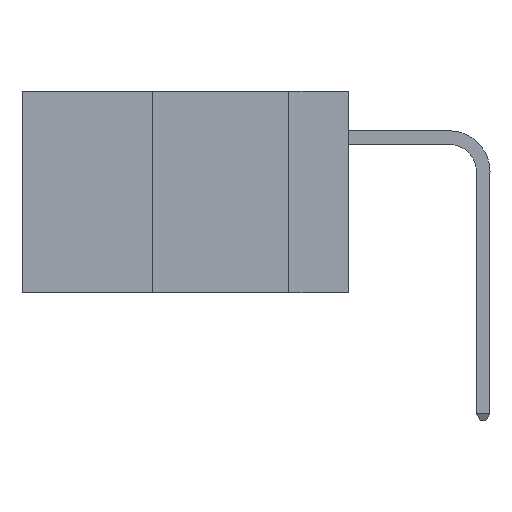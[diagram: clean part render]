
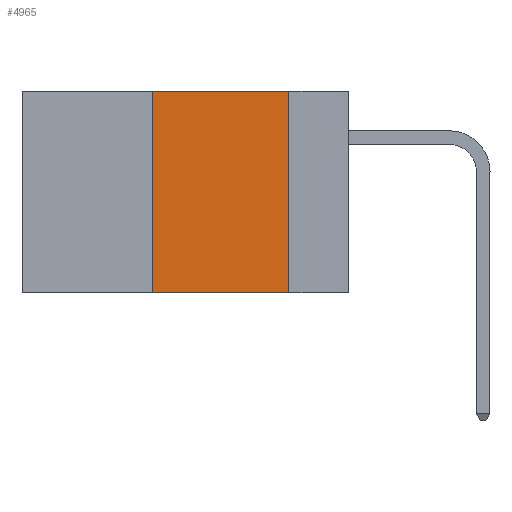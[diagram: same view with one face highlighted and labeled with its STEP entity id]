
A CAD part, left-side view. The second image highlights one B-rep face of the part: STEP entity #4965.
In plain terms, the highlighted planar face has unit normal (-1, 0, 0).
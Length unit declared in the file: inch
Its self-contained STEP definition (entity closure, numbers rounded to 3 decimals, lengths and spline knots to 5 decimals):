
#364 = EDGE_CURVE ( 'NONE', #6327, #7623, #7117, .T. ) ;
#445 = LINE ( 'NONE', #7259, #2283 ) ;
#888 = VECTOR ( 'NONE', #7565, 39.37008 ) ;
#1232 = PLANE ( 'NONE',  #2368 ) ;
#1266 = ORIENTED_EDGE ( 'NONE', *, *, #3956, .F. ) ;
#1365 = EDGE_CURVE ( 'NONE', #6327, #9292, #6985, .T. ) ;
#2129 = DIRECTION ( 'NONE',  ( 1., 0., 0. ) ) ;
#2200 = CARTESIAN_POINT ( 'NONE',  ( 0., 0.36, 0. ) ) ;
#2283 = VECTOR ( 'NONE', #10680, 39.37008 ) ;
#2368 = AXIS2_PLACEMENT_3D ( 'NONE', #7469, #2129, #8333 ) ;
#3110 = CARTESIAN_POINT ( 'NONE',  ( 0., 0.36, 0. ) ) ;
#3817 = DIRECTION ( 'NONE',  ( 0., -1., 0. ) ) ;
#3914 = ORIENTED_EDGE ( 'NONE', *, *, #1365, .F. ) ;
#3925 = ORIENTED_EDGE ( 'NONE', *, *, #9059, .F. ) ;
#3956 = EDGE_CURVE ( 'NONE', #9292, #4129, #8002, .T. ) ;
#4004 = CARTESIAN_POINT ( 'NONE',  ( 0., 0.6, 0. ) ) ;
#4129 = VERTEX_POINT ( 'NONE', #5207 ) ;
#4965 = ADVANCED_FACE ( 'NONE', ( #8970 ), #1232, .F. ) ;
#5207 = CARTESIAN_POINT ( 'NONE',  ( 0., 0.11, 0. ) ) ;
#5246 = EDGE_LOOP ( 'NONE', ( #3925, #1266, #3914, #5788 ) ) ;
#5788 = ORIENTED_EDGE ( 'NONE', *, *, #364, .T. ) ;
#6327 = VERTEX_POINT ( 'NONE', #9562 ) ;
#6985 = LINE ( 'NONE', #2200, #11247 ) ;
#7117 = LINE ( 'NONE', #8646, #11382 ) ;
#7259 = CARTESIAN_POINT ( 'NONE',  ( 0., 0.11, 0. ) ) ;
#7469 = CARTESIAN_POINT ( 'NONE',  ( 0., 0.6, 0. ) ) ;
#7565 = DIRECTION ( 'NONE',  ( 0., -1., 0. ) ) ;
#7623 = VERTEX_POINT ( 'NONE', #10842 ) ;
#8002 = LINE ( 'NONE', #4004, #888 ) ;
#8333 = DIRECTION ( 'NONE',  ( 0., 0., -1. ) ) ;
#8400 = DIRECTION ( 'NONE',  ( 0., 0., 1. ) ) ;
#8646 = CARTESIAN_POINT ( 'NONE',  ( 0., 0.6, -0.37 ) ) ;
#8970 = FACE_OUTER_BOUND ( 'NONE', #5246, .T. ) ;
#9059 = EDGE_CURVE ( 'NONE', #4129, #7623, #445, .T. ) ;
#9292 = VERTEX_POINT ( 'NONE', #3110 ) ;
#9562 = CARTESIAN_POINT ( 'NONE',  ( 0., 0.36, -0.37 ) ) ;
#10680 = DIRECTION ( 'NONE',  ( 0., 0., -1. ) ) ;
#10842 = CARTESIAN_POINT ( 'NONE',  ( 0., 0.11, -0.37 ) ) ;
#11247 = VECTOR ( 'NONE', #8400, 39.37008 ) ;
#11382 = VECTOR ( 'NONE', #3817, 39.37008 ) ;
